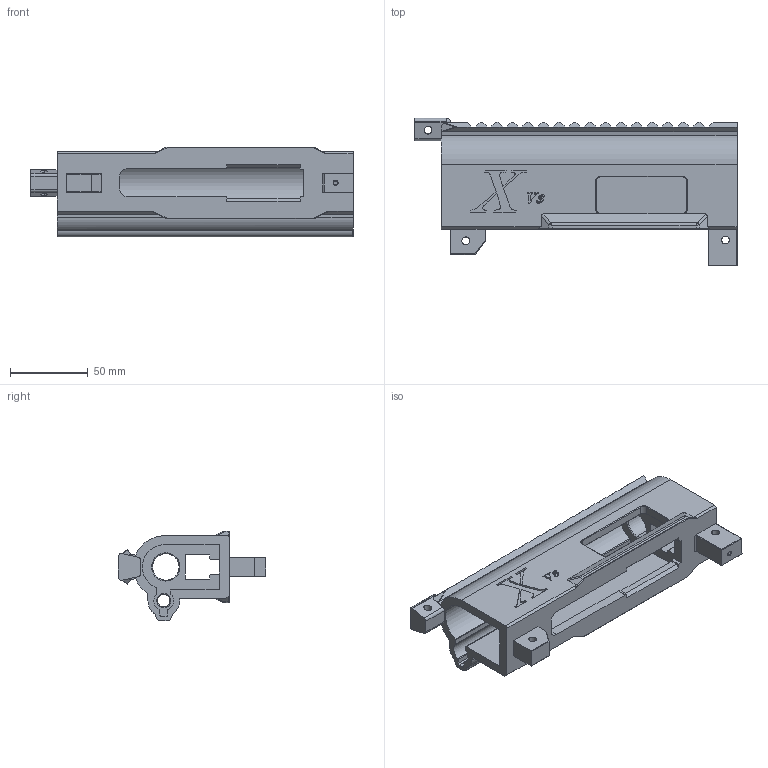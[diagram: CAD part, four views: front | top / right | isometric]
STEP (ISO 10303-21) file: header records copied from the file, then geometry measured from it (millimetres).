
FILE_DESCRIPTION (( 'STEP AP203' ), '1' );
FILE_NAME ('MOD9_V3_Upper.STEP', '2020-12-29T05:04:03', ( '' ), ( '' ), 'SwSTEP 2.0', 'SolidWorks 2019', '' );
FILE_SCHEMA (( 'CONFIG_CONTROL_DESIGN' ));
Length unit declared in the file: millimetre
Products named in the file (1): MOD9_V3_Upper
Bounding box: 207.36 x 94.9 x 57.79 mm (x, y, z)
Volume: 241466.7 mm3; surface area: 83381.9 mm2
Topology: 1 solids, 2 shells, 488 faces, 1281 edges, 808 vertices
Faces by surface type: plane 259, bspline 117, cylinder 88, cone 24
Entity records: 16501 total; most frequent: CARTESIAN_POINT 5242, ORIENTED_EDGE 2558, DIRECTION 1897, EDGE_CURVE 1279, LINE 857, VECTOR 857, VERTEX_POINT 808, AXIS2_PLACEMENT_3D 520
